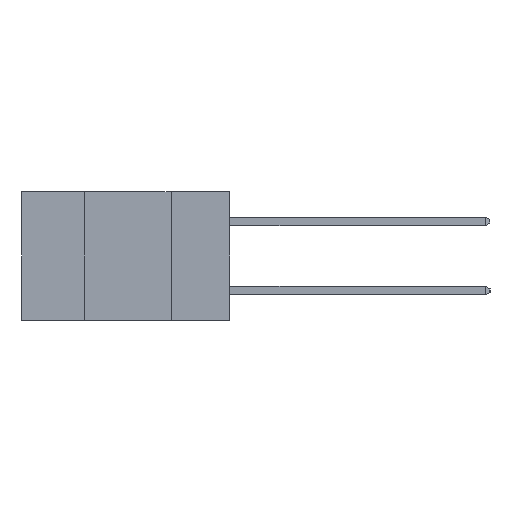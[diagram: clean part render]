
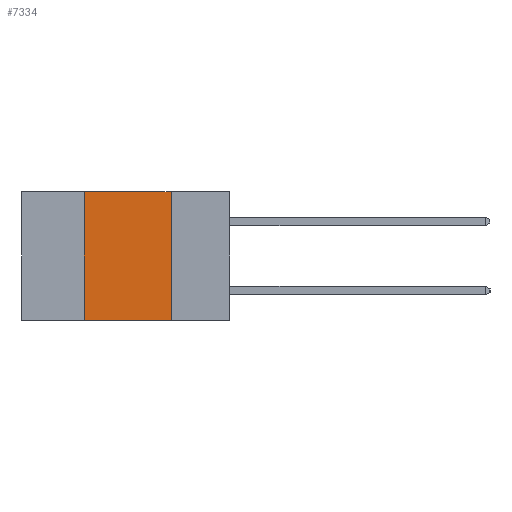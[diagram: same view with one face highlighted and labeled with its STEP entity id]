
A CAD part, left-side view. The second image highlights one B-rep face of the part: STEP entity #7334.
In plain terms, the highlighted planar face has unit normal (-1, 0, 0).
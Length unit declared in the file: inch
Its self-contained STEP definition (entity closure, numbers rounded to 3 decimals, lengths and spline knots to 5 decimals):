
#222 = DIRECTION ( 'NONE',  ( 0., 0., -1. ) ) ;
#479 = FACE_OUTER_BOUND ( 'NONE', #9932, .T. ) ;
#1035 = CARTESIAN_POINT ( 'NONE',  ( 0., 0.17, -0.37 ) ) ;
#1141 = CARTESIAN_POINT ( 'NONE',  ( 0., 0.42, 0. ) ) ;
#1195 = CARTESIAN_POINT ( 'NONE',  ( 0., 0.6, -0.37 ) ) ;
#1263 = DIRECTION ( 'NONE',  ( 0., -1., 0. ) ) ;
#1390 = ORIENTED_EDGE ( 'NONE', *, *, #9498, .T. ) ;
#1923 = VECTOR ( 'NONE', #2901, 39.37008 ) ;
#2281 = CARTESIAN_POINT ( 'NONE',  ( 0., 0.42, -0.37 ) ) ;
#2331 = DIRECTION ( 'NONE',  ( 0., 0., -1. ) ) ;
#2340 = VERTEX_POINT ( 'NONE', #6407 ) ;
#2349 = DIRECTION ( 'NONE',  ( 1., 0., 0. ) ) ;
#2375 = PLANE ( 'NONE',  #2472 ) ;
#2390 = CARTESIAN_POINT ( 'NONE',  ( 0., 0.6, 0. ) ) ;
#2472 = AXIS2_PLACEMENT_3D ( 'NONE', #2390, #2349, #2331 ) ;
#2803 = EDGE_CURVE ( 'NONE', #5878, #2340, #8535, .T. ) ;
#2901 = DIRECTION ( 'NONE',  ( 0., -1., 0. ) ) ;
#3026 = ORIENTED_EDGE ( 'NONE', *, *, #2803, .F. ) ;
#3203 = VECTOR ( 'NONE', #222, 39.37008 ) ;
#3445 = EDGE_CURVE ( 'NONE', #11425, #9500, #8222, .T. ) ;
#3708 = LINE ( 'NONE', #1195, #9610 ) ;
#4645 = LINE ( 'NONE', #8908, #1923 ) ;
#5722 = ORIENTED_EDGE ( 'NONE', *, *, #10455, .F. ) ;
#5878 = VERTEX_POINT ( 'NONE', #9525 ) ;
#6407 = CARTESIAN_POINT ( 'NONE',  ( 0., 0.17, -0.37 ) ) ;
#7334 = ADVANCED_FACE ( 'NONE', ( #479 ), #2375, .F. ) ;
#7603 = CARTESIAN_POINT ( 'NONE',  ( 0., 0.42, -0.37 ) ) ;
#7806 = DIRECTION ( 'NONE',  ( 0., 0., 1. ) ) ;
#8222 = LINE ( 'NONE', #7603, #12509 ) ;
#8535 = LINE ( 'NONE', #1035, #3203 ) ;
#8908 = CARTESIAN_POINT ( 'NONE',  ( 0., 0.6, 0. ) ) ;
#9498 = EDGE_CURVE ( 'NONE', #11425, #2340, #3708, .T. ) ;
#9500 = VERTEX_POINT ( 'NONE', #1141 ) ;
#9525 = CARTESIAN_POINT ( 'NONE',  ( 0., 0.17, 0. ) ) ;
#9610 = VECTOR ( 'NONE', #1263, 39.37008 ) ;
#9932 = EDGE_LOOP ( 'NONE', ( #3026, #5722, #11443, #1390 ) ) ;
#10455 = EDGE_CURVE ( 'NONE', #9500, #5878, #4645, .T. ) ;
#11425 = VERTEX_POINT ( 'NONE', #2281 ) ;
#11443 = ORIENTED_EDGE ( 'NONE', *, *, #3445, .F. ) ;
#12509 = VECTOR ( 'NONE', #7806, 39.37008 ) ;
